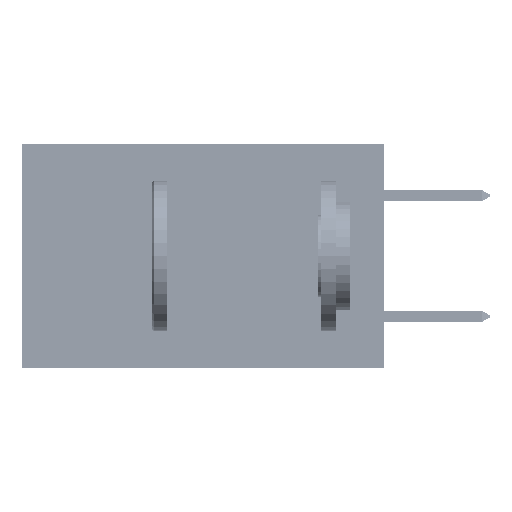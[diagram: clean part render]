
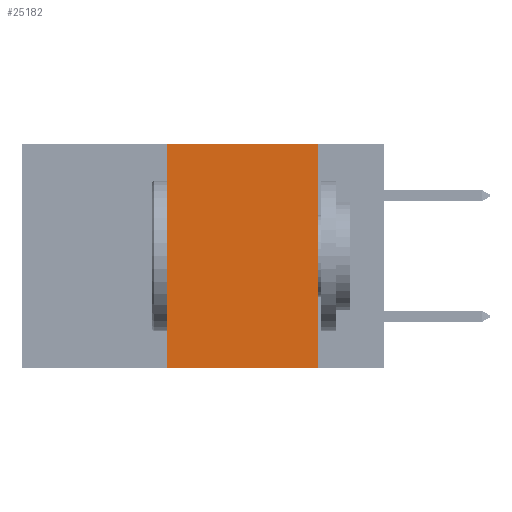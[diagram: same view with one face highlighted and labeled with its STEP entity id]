
A CAD part, left-side view. The second image highlights one B-rep face of the part: STEP entity #25182.
In plain terms, the highlighted planar face has unit normal (-1, 0, 0).
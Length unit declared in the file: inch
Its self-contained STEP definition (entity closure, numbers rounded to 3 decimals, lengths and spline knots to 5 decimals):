
#6027 = VERTEX_POINT ( 'NONE', #27120 ) ;
#7374 = CARTESIAN_POINT ( 'NONE',  ( 0., 0.6, 0. ) ) ;
#7681 = VERTEX_POINT ( 'NONE', #30696 ) ;
#8518 = VECTOR ( 'NONE', #35644, 39.37008 ) ;
#10593 = CARTESIAN_POINT ( 'NONE',  ( 0., 0.36, 0. ) ) ;
#14079 = AXIS2_PLACEMENT_3D ( 'NONE', #7374, #49636, #34042 ) ;
#14454 = ORIENTED_EDGE ( 'NONE', *, *, #16088, .T. ) ;
#15762 = CARTESIAN_POINT ( 'NONE',  ( 0., 0.6, -0.37 ) ) ;
#15885 = LINE ( 'NONE', #10593, #36373 ) ;
#16088 = EDGE_CURVE ( 'NONE', #7681, #35970, #18329, .T. ) ;
#16434 = CARTESIAN_POINT ( 'NONE',  ( 0., 0.6, 0. ) ) ;
#17852 = ORIENTED_EDGE ( 'NONE', *, *, #34927, .F. ) ;
#18329 = LINE ( 'NONE', #15762, #37620 ) ;
#20289 = DIRECTION ( 'NONE',  ( 0., -1., 0. ) ) ;
#23891 = ORIENTED_EDGE ( 'NONE', *, *, #34102, .F. ) ;
#25182 = ADVANCED_FACE ( 'NONE', ( #27082 ), #34553, .F. ) ;
#26042 = EDGE_LOOP ( 'NONE', ( #23891, #26302, #17852, #14454 ) ) ;
#26302 = ORIENTED_EDGE ( 'NONE', *, *, #45425, .F. ) ;
#27082 = FACE_OUTER_BOUND ( 'NONE', #26042, .T. ) ;
#27120 = CARTESIAN_POINT ( 'NONE',  ( 0., 0.11, 0. ) ) ;
#29102 = LINE ( 'NONE', #16434, #8518 ) ;
#30696 = CARTESIAN_POINT ( 'NONE',  ( 0., 0.36, -0.37 ) ) ;
#32168 = VERTEX_POINT ( 'NONE', #36313 ) ;
#34042 = DIRECTION ( 'NONE',  ( 0., 0., -1. ) ) ;
#34102 = EDGE_CURVE ( 'NONE', #6027, #35970, #45489, .T. ) ;
#34553 = PLANE ( 'NONE',  #14079 ) ;
#34927 = EDGE_CURVE ( 'NONE', #7681, #32168, #15885, .T. ) ;
#35644 = DIRECTION ( 'NONE',  ( 0., -1., 0. ) ) ;
#35970 = VERTEX_POINT ( 'NONE', #43448 ) ;
#36313 = CARTESIAN_POINT ( 'NONE',  ( 0., 0.36, 0. ) ) ;
#36373 = VECTOR ( 'NONE', #45246, 39.37008 ) ;
#37620 = VECTOR ( 'NONE', #20289, 39.37008 ) ;
#41327 = VECTOR ( 'NONE', #48707, 39.37008 ) ;
#43448 = CARTESIAN_POINT ( 'NONE',  ( 0., 0.11, -0.37 ) ) ;
#45246 = DIRECTION ( 'NONE',  ( 0., 0., 1. ) ) ;
#45425 = EDGE_CURVE ( 'NONE', #32168, #6027, #29102, .T. ) ;
#45489 = LINE ( 'NONE', #49056, #41327 ) ;
#48707 = DIRECTION ( 'NONE',  ( 0., 0., -1. ) ) ;
#49056 = CARTESIAN_POINT ( 'NONE',  ( 0., 0.11, 0. ) ) ;
#49636 = DIRECTION ( 'NONE',  ( 1., 0., 0. ) ) ;
